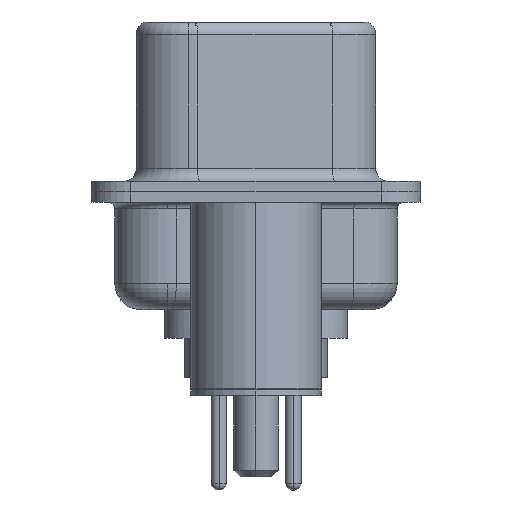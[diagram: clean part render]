
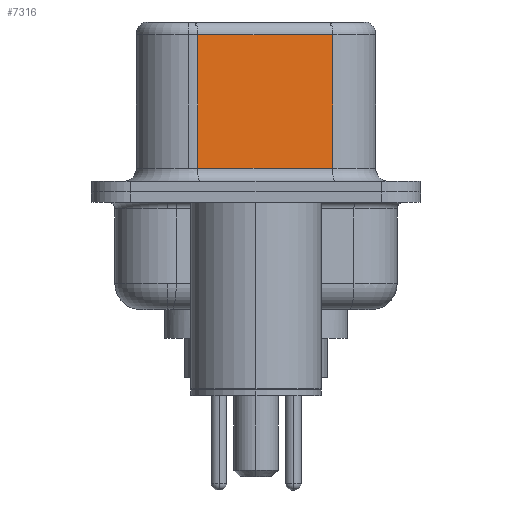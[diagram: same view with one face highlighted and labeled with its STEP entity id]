
A CAD part, left-side view. The second image highlights one B-rep face of the part: STEP entity #7316.
In plain terms, the highlighted planar face has unit normal (-0.985, -0.174, 0).
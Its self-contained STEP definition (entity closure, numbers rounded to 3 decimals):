
#579 = CARTESIAN_POINT ( 'NONE',  ( 4.58, -2.927, 0.9 ) ) ;
#2347 = CARTESIAN_POINT ( 'NONE',  ( 4.58, -2.927, 0.9 ) ) ;
#3004 = ORIENTED_EDGE ( 'NONE', *, *, #10050, .F. ) ;
#3484 = VERTEX_POINT ( 'NONE', #2347 ) ;
#3768 = CARTESIAN_POINT ( 'NONE',  ( 4.58, -2.927, 6.02 ) ) ;
#5672 = ORIENTED_EDGE ( 'NONE', *, *, #20264, .T. ) ;
#5918 = ORIENTED_EDGE ( 'NONE', *, *, #14202, .T. ) ;
#6214 = DIRECTION ( 'NONE',  ( 0.985, 0.174, 0. ) ) ;
#6415 = VERTEX_POINT ( 'NONE', #23996 ) ;
#6422 = DIRECTION ( 'NONE',  ( 0., 0., -1. ) ) ;
#6820 = VECTOR ( 'NONE', #6422, 1000. ) ;
#7316 = ADVANCED_FACE ( 'NONE', ( #20565 ), #12279, .F. ) ;
#7567 = VERTEX_POINT ( 'NONE', #13163 ) ;
#9893 = LINE ( 'NONE', #579, #25794 ) ;
#10050 = EDGE_CURVE ( 'NONE', #6415, #3484, #13653, .T. ) ;
#10759 = DIRECTION ( 'NONE',  ( 0., 0., -1. ) ) ;
#12279 = PLANE ( 'NONE',  #26490 ) ;
#12374 = VECTOR ( 'NONE', #18259, 1000. ) ;
#12838 = CARTESIAN_POINT ( 'NONE',  ( 3.67, 2.233, 6.52 ) ) ;
#13072 = DIRECTION ( 'NONE',  ( 0.174, -0.985, 0. ) ) ;
#13163 = CARTESIAN_POINT ( 'NONE',  ( 3.67, 2.233, 0.9 ) ) ;
#13653 = LINE ( 'NONE', #18837, #6820 ) ;
#14202 = EDGE_CURVE ( 'NONE', #7567, #3484, #9893, .T. ) ;
#15742 = EDGE_CURVE ( 'NONE', #6415, #21263, #23472, .T. ) ;
#18259 = DIRECTION ( 'NONE',  ( -0.174, 0.985, 0. ) ) ;
#18794 = EDGE_LOOP ( 'NONE', ( #3004, #20641, #5672, #5918 ) ) ;
#18837 = CARTESIAN_POINT ( 'NONE',  ( 4.58, -2.927, 6.52 ) ) ;
#20023 = LINE ( 'NONE', #12838, #23628 ) ;
#20162 = CARTESIAN_POINT ( 'NONE',  ( 3.67, 2.233, 6.02 ) ) ;
#20255 = CARTESIAN_POINT ( 'NONE',  ( 4.58, -2.927, 6.52 ) ) ;
#20264 = EDGE_CURVE ( 'NONE', #21263, #7567, #20023, .T. ) ;
#20565 = FACE_OUTER_BOUND ( 'NONE', #18794, .T. ) ;
#20641 = ORIENTED_EDGE ( 'NONE', *, *, #15742, .T. ) ;
#20759 = DIRECTION ( 'NONE',  ( -0.174, 0.985, 0. ) ) ;
#21263 = VERTEX_POINT ( 'NONE', #20162 ) ;
#23472 = LINE ( 'NONE', #3768, #12374 ) ;
#23628 = VECTOR ( 'NONE', #10759, 1000. ) ;
#23996 = CARTESIAN_POINT ( 'NONE',  ( 4.58, -2.927, 6.02 ) ) ;
#25794 = VECTOR ( 'NONE', #13072, 1000. ) ;
#26490 = AXIS2_PLACEMENT_3D ( 'NONE', #20255, #6214, #20759 ) ;
